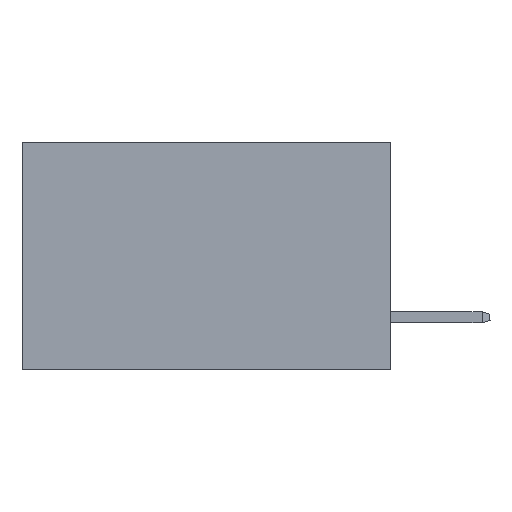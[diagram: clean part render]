
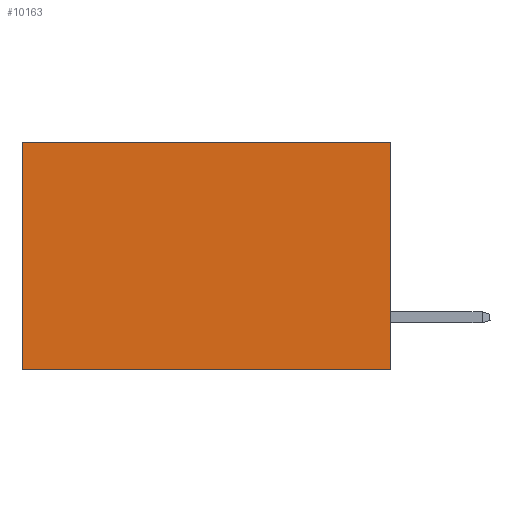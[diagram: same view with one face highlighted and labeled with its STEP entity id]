
A CAD part, left-side view. The second image highlights one B-rep face of the part: STEP entity #10163.
In plain terms, the highlighted planar face has unit normal (-1, 0, 0).
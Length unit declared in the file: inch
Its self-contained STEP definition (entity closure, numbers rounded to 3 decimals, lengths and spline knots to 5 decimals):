
#547 = CARTESIAN_POINT ( 'NONE',  ( 0.2875, 0., 0. ) ) ;
#821 = VERTEX_POINT ( 'NONE', #14957 ) ;
#1164 = EDGE_CURVE ( 'NONE', #11673, #4334, #5881, .T. ) ;
#1265 = LINE ( 'NONE', #13952, #12662 ) ;
#1760 = VECTOR ( 'NONE', #3029, 39.37008 ) ;
#2793 = CARTESIAN_POINT ( 'NONE',  ( 0.2875, 0.6, -0.37 ) ) ;
#2997 = EDGE_LOOP ( 'NONE', ( #6682, #16139, #4554, #17557 ) ) ;
#3029 = DIRECTION ( 'NONE',  ( 0., 0., -1. ) ) ;
#3588 = AXIS2_PLACEMENT_3D ( 'NONE', #7508, #11797, #17502 ) ;
#3758 = FACE_OUTER_BOUND ( 'NONE', #2997, .T. ) ;
#4334 = VERTEX_POINT ( 'NONE', #2793 ) ;
#4554 = ORIENTED_EDGE ( 'NONE', *, *, #6629, .F. ) ;
#4824 = PLANE ( 'NONE',  #3588 ) ;
#5332 = DIRECTION ( 'NONE',  ( 0., 1., 0. ) ) ;
#5756 = EDGE_CURVE ( 'NONE', #821, #4334, #14692, .T. ) ;
#5881 = LINE ( 'NONE', #14372, #12979 ) ;
#6554 = VERTEX_POINT ( 'NONE', #547 ) ;
#6629 = EDGE_CURVE ( 'NONE', #6554, #11673, #1265, .T. ) ;
#6682 = ORIENTED_EDGE ( 'NONE', *, *, #5756, .T. ) ;
#7508 = CARTESIAN_POINT ( 'NONE',  ( 0.2875, 0., 0. ) ) ;
#7735 = EDGE_CURVE ( 'NONE', #6554, #821, #10610, .T. ) ;
#8129 = CARTESIAN_POINT ( 'NONE',  ( 0.2875, 0., 0. ) ) ;
#8536 = DIRECTION ( 'NONE',  ( 0., 1., 0. ) ) ;
#9686 = CARTESIAN_POINT ( 'NONE',  ( 0.2875, 0., -0.37 ) ) ;
#10163 = ADVANCED_FACE ( 'NONE', ( #3758 ), #4824, .F. ) ;
#10610 = LINE ( 'NONE', #8129, #16577 ) ;
#11673 = VERTEX_POINT ( 'NONE', #9686 ) ;
#11797 = DIRECTION ( 'NONE',  ( 1., 0., 0. ) ) ;
#12662 = VECTOR ( 'NONE', #15368, 39.37008 ) ;
#12979 = VECTOR ( 'NONE', #8536, 39.37008 ) ;
#13952 = CARTESIAN_POINT ( 'NONE',  ( 0.2875, 0., 0. ) ) ;
#14372 = CARTESIAN_POINT ( 'NONE',  ( 0.2875, 0., -0.37 ) ) ;
#14511 = CARTESIAN_POINT ( 'NONE',  ( 0.2875, 0.6, 0. ) ) ;
#14692 = LINE ( 'NONE', #14511, #1760 ) ;
#14957 = CARTESIAN_POINT ( 'NONE',  ( 0.2875, 0.6, 0. ) ) ;
#15368 = DIRECTION ( 'NONE',  ( 0., 0., -1. ) ) ;
#16139 = ORIENTED_EDGE ( 'NONE', *, *, #1164, .F. ) ;
#16577 = VECTOR ( 'NONE', #5332, 39.37008 ) ;
#17502 = DIRECTION ( 'NONE',  ( 0., 0., -1. ) ) ;
#17557 = ORIENTED_EDGE ( 'NONE', *, *, #7735, .T. ) ;
